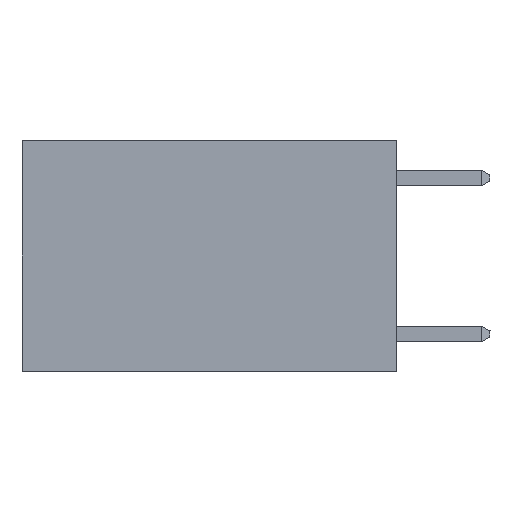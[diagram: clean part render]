
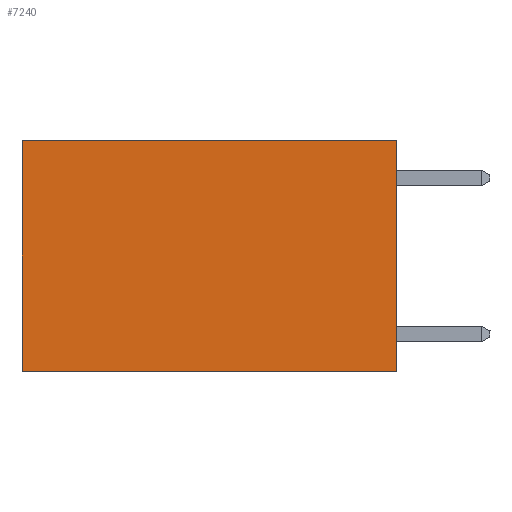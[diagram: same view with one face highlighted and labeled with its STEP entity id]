
A CAD part, left-side view. The second image highlights one B-rep face of the part: STEP entity #7240.
In plain terms, the highlighted planar face has unit normal (-1, 0, 0).
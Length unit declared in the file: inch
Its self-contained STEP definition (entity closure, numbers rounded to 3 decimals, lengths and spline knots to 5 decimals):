
#527 = DIRECTION ( 'NONE',  ( 0., 0., -1. ) ) ;
#686 = LINE ( 'NONE', #2377, #4068 ) ;
#1096 = ORIENTED_EDGE ( 'NONE', *, *, #9753, .F. ) ;
#1262 = LINE ( 'NONE', #4900, #9147 ) ;
#1520 = CARTESIAN_POINT ( 'NONE',  ( 0.2625, 0., 0. ) ) ;
#1842 = ORIENTED_EDGE ( 'NONE', *, *, #6171, .T. ) ;
#2179 = LINE ( 'NONE', #5171, #8346 ) ;
#2329 = DIRECTION ( 'NONE',  ( 0., 0., -1. ) ) ;
#2377 = CARTESIAN_POINT ( 'NONE',  ( 0.2625, 0., 0. ) ) ;
#2499 = VECTOR ( 'NONE', #3262, 39.37008 ) ;
#2978 = VERTEX_POINT ( 'NONE', #1520 ) ;
#3010 = EDGE_CURVE ( 'NONE', #2978, #5070, #686, .T. ) ;
#3130 = ORIENTED_EDGE ( 'NONE', *, *, #3010, .F. ) ;
#3262 = DIRECTION ( 'NONE',  ( 0., 1., 0. ) ) ;
#3294 = CARTESIAN_POINT ( 'NONE',  ( 0.2625, 0.6, -0.37 ) ) ;
#3661 = CARTESIAN_POINT ( 'NONE',  ( 0.2625, 0.6, 0. ) ) ;
#3835 = CARTESIAN_POINT ( 'NONE',  ( 0.2625, 0., 0. ) ) ;
#4068 = VECTOR ( 'NONE', #4722, 39.37008 ) ;
#4529 = EDGE_LOOP ( 'NONE', ( #9009, #1096, #3130, #1842 ) ) ;
#4722 = DIRECTION ( 'NONE',  ( 0., 0., -1. ) ) ;
#4806 = LINE ( 'NONE', #7929, #2499 ) ;
#4900 = CARTESIAN_POINT ( 'NONE',  ( 0.2625, 0., 0. ) ) ;
#5070 = VERTEX_POINT ( 'NONE', #7589 ) ;
#5171 = CARTESIAN_POINT ( 'NONE',  ( 0.2625, 0.6, 0. ) ) ;
#5417 = PLANE ( 'NONE',  #6882 ) ;
#5694 = DIRECTION ( 'NONE',  ( 0., 1., 0. ) ) ;
#5718 = FACE_OUTER_BOUND ( 'NONE', #4529, .T. ) ;
#6171 = EDGE_CURVE ( 'NONE', #2978, #9414, #1262, .T. ) ;
#6882 = AXIS2_PLACEMENT_3D ( 'NONE', #3835, #6991, #2329 ) ;
#6991 = DIRECTION ( 'NONE',  ( 1., 0., 0. ) ) ;
#7240 = ADVANCED_FACE ( 'NONE', ( #5718 ), #5417, .F. ) ;
#7589 = CARTESIAN_POINT ( 'NONE',  ( 0.2625, 0., -0.37 ) ) ;
#7929 = CARTESIAN_POINT ( 'NONE',  ( 0.2625, 0., -0.37 ) ) ;
#8346 = VECTOR ( 'NONE', #527, 39.37008 ) ;
#8712 = EDGE_CURVE ( 'NONE', #9414, #9769, #2179, .T. ) ;
#9009 = ORIENTED_EDGE ( 'NONE', *, *, #8712, .T. ) ;
#9147 = VECTOR ( 'NONE', #5694, 39.37008 ) ;
#9414 = VERTEX_POINT ( 'NONE', #3661 ) ;
#9753 = EDGE_CURVE ( 'NONE', #5070, #9769, #4806, .T. ) ;
#9769 = VERTEX_POINT ( 'NONE', #3294 ) ;
